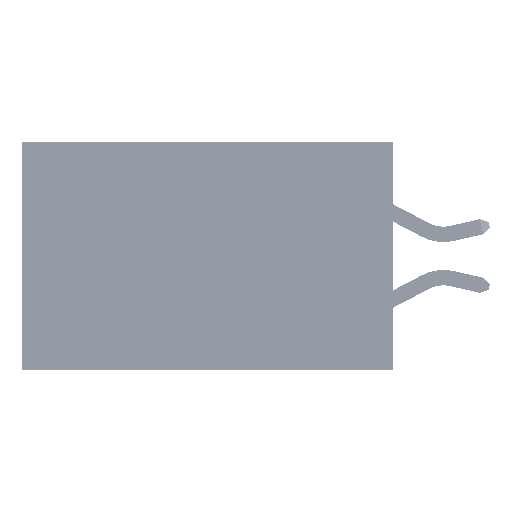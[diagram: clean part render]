
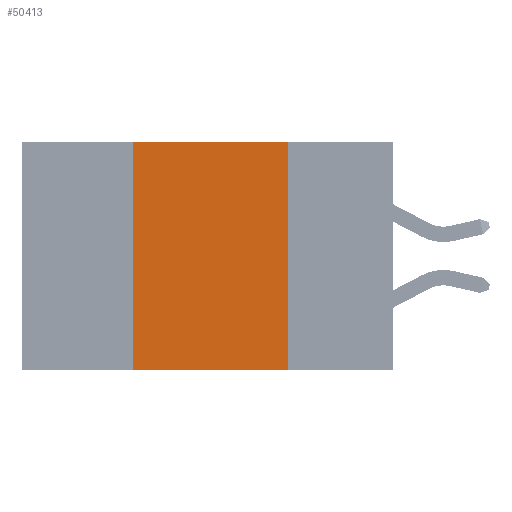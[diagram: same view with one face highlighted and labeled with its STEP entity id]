
A CAD part, left-side view. The second image highlights one B-rep face of the part: STEP entity #50413.
In plain terms, the highlighted planar face has unit normal (-1, 0, 0).
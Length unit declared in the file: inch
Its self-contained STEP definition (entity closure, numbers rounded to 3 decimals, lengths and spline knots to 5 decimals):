
#3132 = EDGE_CURVE ( 'NONE', #16152, #31303, #17433, .T. ) ;
#4166 = VECTOR ( 'NONE', #15630, 39.37008 ) ;
#6250 = ORIENTED_EDGE ( 'NONE', *, *, #3132, .F. ) ;
#6332 = ORIENTED_EDGE ( 'NONE', *, *, #11305, .T. ) ;
#6393 = VECTOR ( 'NONE', #35397, 39.37008 ) ;
#6828 = DIRECTION ( 'NONE',  ( 1., 0., 0. ) ) ;
#8136 = FACE_OUTER_BOUND ( 'NONE', #9847, .T. ) ;
#8473 = AXIS2_PLACEMENT_3D ( 'NONE', #26951, #6828, #35026 ) ;
#9847 = EDGE_LOOP ( 'NONE', ( #49217, #9880, #6250, #6332 ) ) ;
#9880 = ORIENTED_EDGE ( 'NONE', *, *, #13017, .F. ) ;
#10701 = VERTEX_POINT ( 'NONE', #34307 ) ;
#10898 = CARTESIAN_POINT ( 'NONE',  ( 0., 0.17, 0. ) ) ;
#11305 = EDGE_CURVE ( 'NONE', #16152, #10701, #14148, .T. ) ;
#11321 = CARTESIAN_POINT ( 'NONE',  ( 0., 0.42, -0.37 ) ) ;
#11507 = LINE ( 'NONE', #25349, #33584 ) ;
#13017 = EDGE_CURVE ( 'NONE', #31303, #25791, #11507, .T. ) ;
#14148 = LINE ( 'NONE', #43079, #16680 ) ;
#14213 = CARTESIAN_POINT ( 'NONE',  ( 0., 0.17, 0. ) ) ;
#15630 = DIRECTION ( 'NONE',  ( 0., 0., 1. ) ) ;
#16152 = VERTEX_POINT ( 'NONE', #11321 ) ;
#16680 = VECTOR ( 'NONE', #30369, 39.37008 ) ;
#17433 = LINE ( 'NONE', #23570, #4166 ) ;
#23570 = CARTESIAN_POINT ( 'NONE',  ( 0., 0.42, 0. ) ) ;
#25349 = CARTESIAN_POINT ( 'NONE',  ( 0., 0.6, 0. ) ) ;
#25785 = CARTESIAN_POINT ( 'NONE',  ( 0., 0.42, 0. ) ) ;
#25791 = VERTEX_POINT ( 'NONE', #14213 ) ;
#26951 = CARTESIAN_POINT ( 'NONE',  ( 0., 0.6, 0. ) ) ;
#29699 = LINE ( 'NONE', #10898, #6393 ) ;
#30369 = DIRECTION ( 'NONE',  ( 0., -1., 0. ) ) ;
#31303 = VERTEX_POINT ( 'NONE', #25785 ) ;
#31490 = PLANE ( 'NONE',  #8473 ) ;
#32015 = EDGE_CURVE ( 'NONE', #25791, #10701, #29699, .T. ) ;
#33584 = VECTOR ( 'NONE', #45410, 39.37008 ) ;
#34307 = CARTESIAN_POINT ( 'NONE',  ( 0., 0.17, -0.37 ) ) ;
#35026 = DIRECTION ( 'NONE',  ( 0., 0., -1. ) ) ;
#35397 = DIRECTION ( 'NONE',  ( 0., 0., -1. ) ) ;
#43079 = CARTESIAN_POINT ( 'NONE',  ( 0., 0.6, -0.37 ) ) ;
#45410 = DIRECTION ( 'NONE',  ( 0., -1., 0. ) ) ;
#49217 = ORIENTED_EDGE ( 'NONE', *, *, #32015, .F. ) ;
#50413 = ADVANCED_FACE ( 'NONE', ( #8136 ), #31490, .F. ) ;
